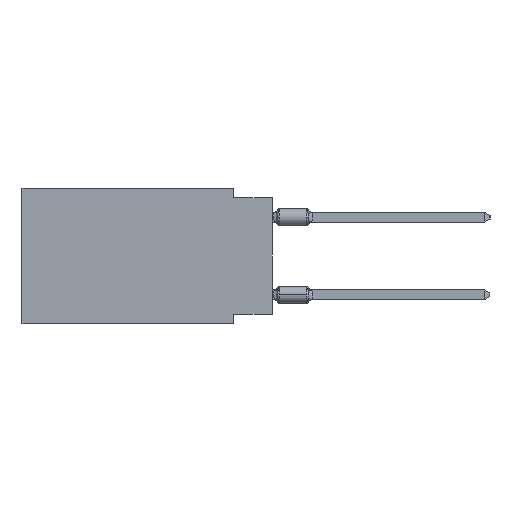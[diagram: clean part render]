
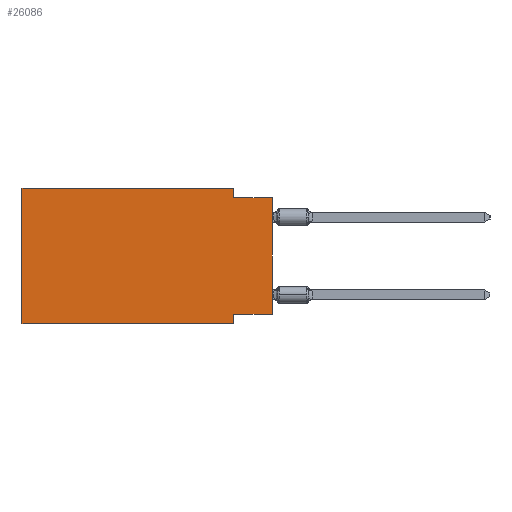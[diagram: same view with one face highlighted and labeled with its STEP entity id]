
A CAD part, left-side view. The second image highlights one B-rep face of the part: STEP entity #26086.
In plain terms, the highlighted planar face has unit normal (-1, 0, 0).
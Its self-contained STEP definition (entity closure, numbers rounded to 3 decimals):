
#479 = CARTESIAN_POINT ( 'NONE',  ( 0., 16.383, -8.89 ) ) ;
#1498 = CARTESIAN_POINT ( 'NONE',  ( 0., 16.383, 0. ) ) ;
#2395 = CARTESIAN_POINT ( 'NONE',  ( 0., 16.383, 0. ) ) ;
#2637 = DIRECTION ( 'NONE',  ( 0., 0., -1. ) ) ;
#2903 = LINE ( 'NONE', #16290, #35169 ) ;
#3111 = LINE ( 'NONE', #32224, #24547 ) ;
#3186 = DIRECTION ( 'NONE',  ( 0., 0., -1. ) ) ;
#3201 = CARTESIAN_POINT ( 'NONE',  ( 0., 2.54, -0.635 ) ) ;
#3259 = FACE_OUTER_BOUND ( 'NONE', #32852, .T. ) ;
#4090 = CARTESIAN_POINT ( 'NONE',  ( 0., 2.54, -8.255 ) ) ;
#4766 = DIRECTION ( 'NONE',  ( 0., 0., -1. ) ) ;
#4896 = VECTOR ( 'NONE', #10271, 1000. ) ;
#5408 = EDGE_CURVE ( 'NONE', #25225, #9804, #2903, .T. ) ;
#5653 = ORIENTED_EDGE ( 'NONE', *, *, #41448, .F. ) ;
#9309 = VECTOR ( 'NONE', #4766, 1000. ) ;
#9529 = VECTOR ( 'NONE', #34808, 1000. ) ;
#9804 = VERTEX_POINT ( 'NONE', #23062 ) ;
#10271 = DIRECTION ( 'NONE',  ( 0., -1., 0. ) ) ;
#10621 = CARTESIAN_POINT ( 'NONE',  ( 0., 2.54, 0. ) ) ;
#10790 = EDGE_CURVE ( 'NONE', #24416, #18825, #21529, .T. ) ;
#11657 = ORIENTED_EDGE ( 'NONE', *, *, #10790, .F. ) ;
#12589 = ORIENTED_EDGE ( 'NONE', *, *, #5408, .T. ) ;
#12686 = VECTOR ( 'NONE', #33820, 1000. ) ;
#13603 = EDGE_CURVE ( 'NONE', #25225, #24416, #3111, .T. ) ;
#14245 = ORIENTED_EDGE ( 'NONE', *, *, #13603, .F. ) ;
#14306 = EDGE_CURVE ( 'NONE', #37530, #18825, #29595, .T. ) ;
#15382 = DIRECTION ( 'NONE',  ( 0., 0., 1. ) ) ;
#16290 = CARTESIAN_POINT ( 'NONE',  ( 0., 0., 0. ) ) ;
#18789 = CARTESIAN_POINT ( 'NONE',  ( 0., 16.383, 0. ) ) ;
#18825 = VERTEX_POINT ( 'NONE', #22471 ) ;
#20701 = VERTEX_POINT ( 'NONE', #2395 ) ;
#21529 = LINE ( 'NONE', #21733, #9309 ) ;
#21733 = CARTESIAN_POINT ( 'NONE',  ( 0., 2.54, -8.89 ) ) ;
#22449 = LINE ( 'NONE', #31618, #9529 ) ;
#22471 = CARTESIAN_POINT ( 'NONE',  ( 0., 2.54, -8.89 ) ) ;
#23062 = CARTESIAN_POINT ( 'NONE',  ( 0., 0., -0.635 ) ) ;
#23549 = LINE ( 'NONE', #10621, #32731 ) ;
#24007 = LINE ( 'NONE', #1498, #12686 ) ;
#24416 = VERTEX_POINT ( 'NONE', #4090 ) ;
#24547 = VECTOR ( 'NONE', #28817, 1000. ) ;
#25125 = CARTESIAN_POINT ( 'NONE',  ( 0., 16.383, 0. ) ) ;
#25225 = VERTEX_POINT ( 'NONE', #28276 ) ;
#25323 = VERTEX_POINT ( 'NONE', #3201 ) ;
#25891 = CARTESIAN_POINT ( 'NONE',  ( 0., 2.54, 0. ) ) ;
#26086 = ADVANCED_FACE ( 'NONE', ( #3259 ), #34957, .F. ) ;
#26210 = CARTESIAN_POINT ( 'NONE',  ( 0., 16.383, -8.89 ) ) ;
#26662 = EDGE_CURVE ( 'NONE', #37530, #20701, #35555, .T. ) ;
#27147 = ORIENTED_EDGE ( 'NONE', *, *, #39937, .F. ) ;
#27167 = ORIENTED_EDGE ( 'NONE', *, *, #14306, .T. ) ;
#28276 = CARTESIAN_POINT ( 'NONE',  ( 0., 0., -8.255 ) ) ;
#28817 = DIRECTION ( 'NONE',  ( 0., 1., 0. ) ) ;
#29240 = DIRECTION ( 'NONE',  ( 0., 0., 1. ) ) ;
#29583 = VERTEX_POINT ( 'NONE', #25891 ) ;
#29595 = LINE ( 'NONE', #479, #4896 ) ;
#30901 = VECTOR ( 'NONE', #15382, 1000. ) ;
#31618 = CARTESIAN_POINT ( 'NONE',  ( 0., 0., -0.635 ) ) ;
#31757 = DIRECTION ( 'NONE',  ( 1., 0., 0. ) ) ;
#32224 = CARTESIAN_POINT ( 'NONE',  ( 0., 0., -8.255 ) ) ;
#32731 = VECTOR ( 'NONE', #3186, 1000. ) ;
#32852 = EDGE_LOOP ( 'NONE', ( #12589, #5653, #34406, #27147, #37103, #27167, #11657, #14245 ) ) ;
#33039 = EDGE_CURVE ( 'NONE', #29583, #25323, #23549, .T. ) ;
#33820 = DIRECTION ( 'NONE',  ( 0., -1., 0. ) ) ;
#34406 = ORIENTED_EDGE ( 'NONE', *, *, #33039, .F. ) ;
#34808 = DIRECTION ( 'NONE',  ( 0., -1., 0. ) ) ;
#34957 = PLANE ( 'NONE',  #37640 ) ;
#35169 = VECTOR ( 'NONE', #29240, 1000. ) ;
#35555 = LINE ( 'NONE', #25125, #30901 ) ;
#37103 = ORIENTED_EDGE ( 'NONE', *, *, #26662, .F. ) ;
#37530 = VERTEX_POINT ( 'NONE', #26210 ) ;
#37640 = AXIS2_PLACEMENT_3D ( 'NONE', #18789, #31757, #2637 ) ;
#39937 = EDGE_CURVE ( 'NONE', #20701, #29583, #24007, .T. ) ;
#41448 = EDGE_CURVE ( 'NONE', #25323, #9804, #22449, .T. ) ;
